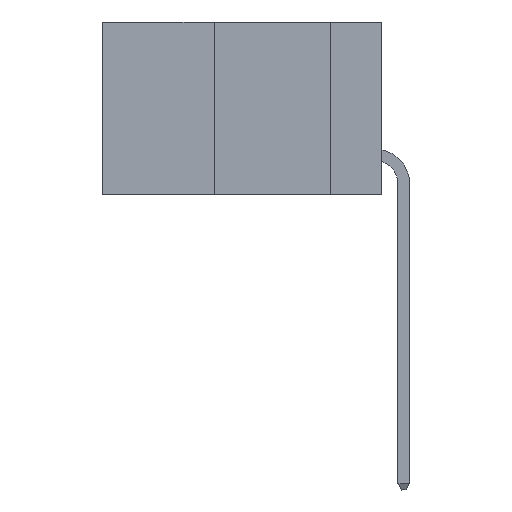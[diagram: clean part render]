
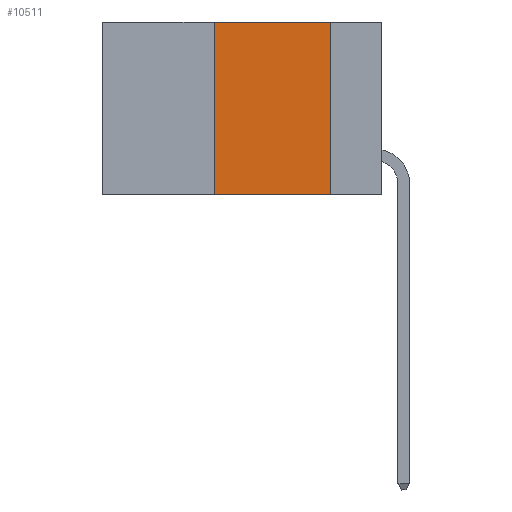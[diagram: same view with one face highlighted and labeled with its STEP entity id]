
A CAD part, left-side view. The second image highlights one B-rep face of the part: STEP entity #10511.
In plain terms, the highlighted planar face has unit normal (-1, 0, 0).
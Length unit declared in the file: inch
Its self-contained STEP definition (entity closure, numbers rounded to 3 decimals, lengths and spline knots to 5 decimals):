
#1157 = VECTOR ( 'NONE', #17589, 39.37008 ) ;
#1698 = DIRECTION ( 'NONE',  ( 0., 0., 1. ) ) ;
#4113 = CARTESIAN_POINT ( 'NONE',  ( 0., 0.36, -0.37 ) ) ;
#4946 = VERTEX_POINT ( 'NONE', #13603 ) ;
#6424 = CARTESIAN_POINT ( 'NONE',  ( 0., 0.36, 0. ) ) ;
#7656 = PLANE ( 'NONE',  #17005 ) ;
#8241 = VECTOR ( 'NONE', #29777, 39.37008 ) ;
#10511 = ADVANCED_FACE ( 'NONE', ( #12139 ), #7656, .F. ) ;
#12026 = VERTEX_POINT ( 'NONE', #23561 ) ;
#12139 = FACE_OUTER_BOUND ( 'NONE', #12231, .T. ) ;
#12231 = EDGE_LOOP ( 'NONE', ( #22773, #26064, #31208, #30366 ) ) ;
#13321 = DIRECTION ( 'NONE',  ( 0., 0., -1. ) ) ;
#13603 = CARTESIAN_POINT ( 'NONE',  ( 0., 0.36, 0. ) ) ;
#14850 = CARTESIAN_POINT ( 'NONE',  ( 0., 0.11, 0. ) ) ;
#14876 = LINE ( 'NONE', #14850, #24838 ) ;
#16056 = LINE ( 'NONE', #17827, #1157 ) ;
#17005 = AXIS2_PLACEMENT_3D ( 'NONE', #26953, #18853, #13321 ) ;
#17589 = DIRECTION ( 'NONE',  ( 0., -1., 0. ) ) ;
#17827 = CARTESIAN_POINT ( 'NONE',  ( 0., 0.6, -0.37 ) ) ;
#18784 = EDGE_CURVE ( 'NONE', #33316, #12026, #16056, .T. ) ;
#18853 = DIRECTION ( 'NONE',  ( 1., 0., 0. ) ) ;
#19227 = CARTESIAN_POINT ( 'NONE',  ( 0., 0.6, 0. ) ) ;
#19570 = VECTOR ( 'NONE', #1698, 39.37008 ) ;
#21241 = LINE ( 'NONE', #6424, #19570 ) ;
#21588 = EDGE_CURVE ( 'NONE', #33316, #4946, #21241, .T. ) ;
#22773 = ORIENTED_EDGE ( 'NONE', *, *, #26421, .F. ) ;
#23561 = CARTESIAN_POINT ( 'NONE',  ( 0., 0.11, -0.37 ) ) ;
#24838 = VECTOR ( 'NONE', #25286, 39.37008 ) ;
#25200 = EDGE_CURVE ( 'NONE', #4946, #29447, #26488, .T. ) ;
#25286 = DIRECTION ( 'NONE',  ( 0., 0., -1. ) ) ;
#26064 = ORIENTED_EDGE ( 'NONE', *, *, #25200, .F. ) ;
#26421 = EDGE_CURVE ( 'NONE', #29447, #12026, #14876, .T. ) ;
#26488 = LINE ( 'NONE', #19227, #8241 ) ;
#26953 = CARTESIAN_POINT ( 'NONE',  ( 0., 0.6, 0. ) ) ;
#27439 = CARTESIAN_POINT ( 'NONE',  ( 0., 0.11, 0. ) ) ;
#29447 = VERTEX_POINT ( 'NONE', #27439 ) ;
#29777 = DIRECTION ( 'NONE',  ( 0., -1., 0. ) ) ;
#30366 = ORIENTED_EDGE ( 'NONE', *, *, #18784, .T. ) ;
#31208 = ORIENTED_EDGE ( 'NONE', *, *, #21588, .F. ) ;
#33316 = VERTEX_POINT ( 'NONE', #4113 ) ;
